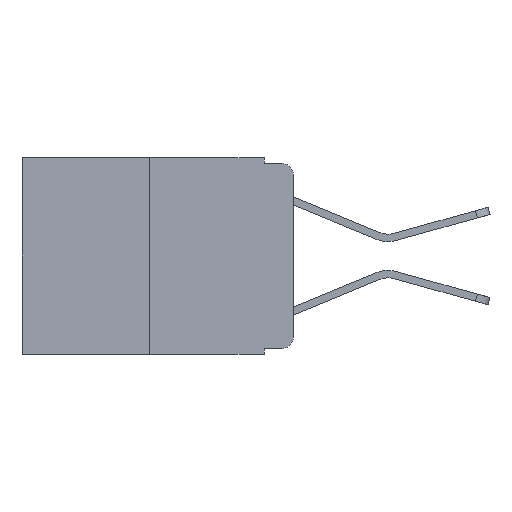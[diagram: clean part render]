
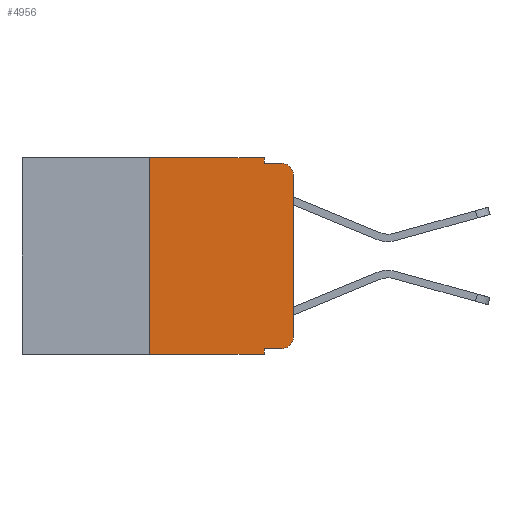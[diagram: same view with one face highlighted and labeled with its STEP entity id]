
A CAD part, left-side view. The second image highlights one B-rep face of the part: STEP entity #4956.
In plain terms, the highlighted planar face has unit normal (-1, 0, 0).
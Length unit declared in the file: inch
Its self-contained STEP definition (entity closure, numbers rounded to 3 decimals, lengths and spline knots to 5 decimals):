
#171 = EDGE_LOOP ( 'NONE', ( #4866, #9920, #12282, #5167, #7711, #10212, #2948, #10503, #663, #3243 ) ) ;
#371 = VERTEX_POINT ( 'NONE', #11555 ) ;
#663 = ORIENTED_EDGE ( 'NONE', *, *, #10704, .T. ) ;
#992 = LINE ( 'NONE', #8032, #3261 ) ;
#1198 = FACE_OUTER_BOUND ( 'NONE', #171, .T. ) ;
#1226 = CARTESIAN_POINT ( 'NONE',  ( 0., 0.02, -0.01 ) ) ;
#1265 = EDGE_CURVE ( 'NONE', #3072, #6324, #10633, .T. ) ;
#1357 = LINE ( 'NONE', #11175, #11130 ) ;
#1369 = VECTOR ( 'NONE', #1752, 39.37008 ) ;
#1493 = DIRECTION ( 'NONE',  ( 0., 0., 1. ) ) ;
#1620 = PLANE ( 'NONE',  #2242 ) ;
#1752 = DIRECTION ( 'NONE',  ( 0., -1., 0. ) ) ;
#1827 = LINE ( 'NONE', #9573, #11263 ) ;
#1957 = DIRECTION ( 'NONE',  ( 0., -1., 0. ) ) ;
#2242 = AXIS2_PLACEMENT_3D ( 'NONE', #11918, #10178, #4492 ) ;
#2287 = VECTOR ( 'NONE', #1957, 39.37008 ) ;
#2741 = CARTESIAN_POINT ( 'NONE',  ( 0., 0.25, -0.343 ) ) ;
#2948 = ORIENTED_EDGE ( 'NONE', *, *, #3573, .T. ) ;
#3072 = VERTEX_POINT ( 'NONE', #3662 ) ;
#3236 = DIRECTION ( 'NONE',  ( 0., -1., 0. ) ) ;
#3243 = ORIENTED_EDGE ( 'NONE', *, *, #10887, .T. ) ;
#3261 = VECTOR ( 'NONE', #3236, 39.37008 ) ;
#3573 = EDGE_CURVE ( 'NONE', #6168, #8345, #3925, .T. ) ;
#3662 = CARTESIAN_POINT ( 'NONE',  ( 0., 0.051, 0. ) ) ;
#3792 = EDGE_CURVE ( 'NONE', #10947, #8345, #1827, .T. ) ;
#3818 = CARTESIAN_POINT ( 'NONE',  ( 0., 0.02, -0.03 ) ) ;
#3925 = LINE ( 'NONE', #10382, #1369 ) ;
#4020 = EDGE_CURVE ( 'NONE', #8283, #6362, #1357, .T. ) ;
#4079 = CARTESIAN_POINT ( 'NONE',  ( 0., 0.25, 0. ) ) ;
#4131 = DIRECTION ( 'NONE',  ( -1., 0., 0. ) ) ;
#4219 = CARTESIAN_POINT ( 'NONE',  ( 0., 0.051, -0.333 ) ) ;
#4400 = DIRECTION ( 'NONE',  ( 0., 0., -1. ) ) ;
#4413 = EDGE_CURVE ( 'NONE', #7403, #3072, #7042, .T. ) ;
#4488 = VECTOR ( 'NONE', #9413, 39.37008 ) ;
#4492 = DIRECTION ( 'NONE',  ( 0., 0., -1. ) ) ;
#4504 = LINE ( 'NONE', #4079, #11667 ) ;
#4673 = EDGE_CURVE ( 'NONE', #6168, #7403, #4504, .T. ) ;
#4785 = DIRECTION ( 'NONE',  ( 0., 0., -1. ) ) ;
#4866 = ORIENTED_EDGE ( 'NONE', *, *, #4020, .T. ) ;
#4956 = ADVANCED_FACE ( 'NONE', ( #1198 ), #1620, .F. ) ;
#5167 = ORIENTED_EDGE ( 'NONE', *, *, #1265, .F. ) ;
#5393 = AXIS2_PLACEMENT_3D ( 'NONE', #3818, #10453, #4785 ) ;
#5835 = CARTESIAN_POINT ( 'NONE',  ( 0., 0.051, -0.01 ) ) ;
#6168 = VERTEX_POINT ( 'NONE', #2741 ) ;
#6324 = VERTEX_POINT ( 'NONE', #5835 ) ;
#6362 = VERTEX_POINT ( 'NONE', #8720 ) ;
#7042 = LINE ( 'NONE', #7504, #4488 ) ;
#7403 = VERTEX_POINT ( 'NONE', #10724 ) ;
#7504 = CARTESIAN_POINT ( 'NONE',  ( 0., 0.473, 0. ) ) ;
#7659 = CARTESIAN_POINT ( 'NONE',  ( 0., 0.051, -0.333 ) ) ;
#7711 = ORIENTED_EDGE ( 'NONE', *, *, #4413, .F. ) ;
#8032 = CARTESIAN_POINT ( 'NONE',  ( 0., 0.051, -0.01 ) ) ;
#8161 = VECTOR ( 'NONE', #4400, 39.37008 ) ;
#8186 = CARTESIAN_POINT ( 'NONE',  ( 0., 0., -0.313 ) ) ;
#8283 = VERTEX_POINT ( 'NONE', #8186 ) ;
#8345 = VERTEX_POINT ( 'NONE', #10276 ) ;
#8558 = VERTEX_POINT ( 'NONE', #1226 ) ;
#8702 = CARTESIAN_POINT ( 'NONE',  ( 0., 0.051, 0. ) ) ;
#8720 = CARTESIAN_POINT ( 'NONE',  ( 0., 0., -0.03 ) ) ;
#8769 = CIRCLE ( 'NONE', #5393, 0.02 ) ;
#8882 = EDGE_CURVE ( 'NONE', #6362, #8558, #8769, .T. ) ;
#9166 = EDGE_CURVE ( 'NONE', #6324, #8558, #992, .T. ) ;
#9413 = DIRECTION ( 'NONE',  ( 0., -1., 0. ) ) ;
#9459 = AXIS2_PLACEMENT_3D ( 'NONE', #9845, #4131, #10756 ) ;
#9573 = CARTESIAN_POINT ( 'NONE',  ( 0., 0.051, 0. ) ) ;
#9772 = DIRECTION ( 'NONE',  ( 0., 0., 1. ) ) ;
#9845 = CARTESIAN_POINT ( 'NONE',  ( 0., 0.02, -0.313 ) ) ;
#9920 = ORIENTED_EDGE ( 'NONE', *, *, #8882, .T. ) ;
#10137 = DIRECTION ( 'NONE',  ( 0., 0., -1. ) ) ;
#10178 = DIRECTION ( 'NONE',  ( 1., 0., 0. ) ) ;
#10212 = ORIENTED_EDGE ( 'NONE', *, *, #4673, .F. ) ;
#10276 = CARTESIAN_POINT ( 'NONE',  ( 0., 0.051, -0.343 ) ) ;
#10304 = CIRCLE ( 'NONE', #9459, 0.02 ) ;
#10382 = CARTESIAN_POINT ( 'NONE',  ( 0., 0.473, -0.343 ) ) ;
#10453 = DIRECTION ( 'NONE',  ( -1., 0., 0. ) ) ;
#10503 = ORIENTED_EDGE ( 'NONE', *, *, #3792, .F. ) ;
#10633 = LINE ( 'NONE', #8702, #8161 ) ;
#10704 = EDGE_CURVE ( 'NONE', #10947, #371, #12233, .T. ) ;
#10724 = CARTESIAN_POINT ( 'NONE',  ( 0., 0.25, 0. ) ) ;
#10756 = DIRECTION ( 'NONE',  ( 0., 0., -1. ) ) ;
#10887 = EDGE_CURVE ( 'NONE', #371, #8283, #10304, .T. ) ;
#10947 = VERTEX_POINT ( 'NONE', #4219 ) ;
#11130 = VECTOR ( 'NONE', #1493, 39.37008 ) ;
#11175 = CARTESIAN_POINT ( 'NONE',  ( 0., 0., 0. ) ) ;
#11263 = VECTOR ( 'NONE', #10137, 39.37008 ) ;
#11555 = CARTESIAN_POINT ( 'NONE',  ( 0., 0.02, -0.333 ) ) ;
#11667 = VECTOR ( 'NONE', #9772, 39.37008 ) ;
#11918 = CARTESIAN_POINT ( 'NONE',  ( 0., 0.473, 0. ) ) ;
#12233 = LINE ( 'NONE', #7659, #2287 ) ;
#12282 = ORIENTED_EDGE ( 'NONE', *, *, #9166, .F. ) ;
